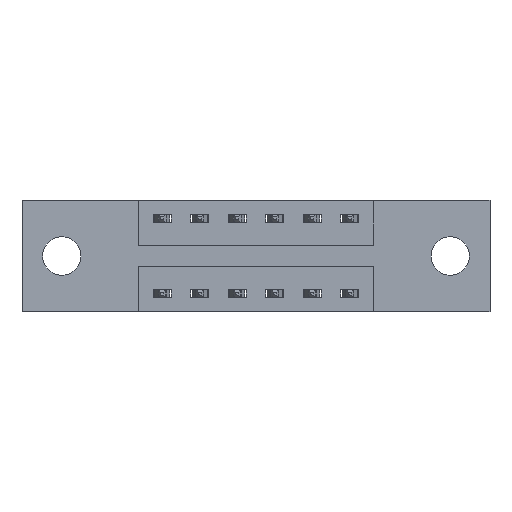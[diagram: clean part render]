
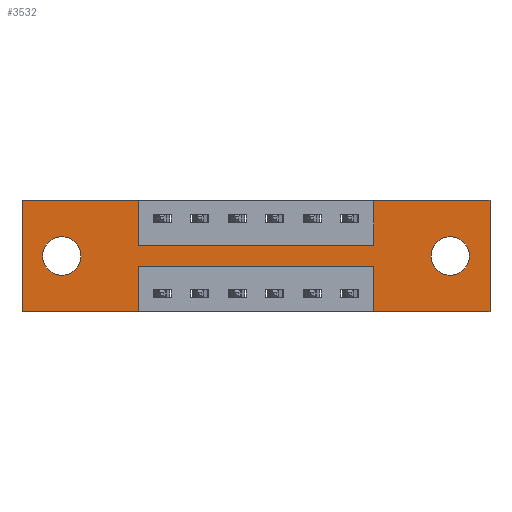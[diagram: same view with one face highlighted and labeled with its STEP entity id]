
A CAD part, front view. The second image highlights one B-rep face of the part: STEP entity #3532.
In plain terms, the highlighted planar face has unit normal (0, -1, 0).
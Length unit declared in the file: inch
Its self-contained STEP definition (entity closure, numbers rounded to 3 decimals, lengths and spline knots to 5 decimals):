
#54 = CARTESIAN_POINT ( 'NONE',  ( 1.1725, 0., 0. ) ) ;
#122 = EDGE_CURVE ( 'NONE', #3930, #1877, #3443, .T. ) ;
#149 = ORIENTED_EDGE ( 'NONE', *, *, #7531, .F. ) ;
#158 = FACE_BOUND ( 'NONE', #3052, .T. ) ;
#201 = CARTESIAN_POINT ( 'NONE',  ( 0.3875, 0., -0.37 ) ) ;
#232 = DIRECTION ( 'NONE',  ( 0., 0., -1. ) ) ;
#447 = CARTESIAN_POINT ( 'NONE',  ( 0.3875, 0., -0.15 ) ) ;
#563 = EDGE_CURVE ( 'NONE', #3608, #4599, #3827, .T. ) ;
#710 = EDGE_CURVE ( 'NONE', #7500, #4958, #1879, .T. ) ;
#736 = CARTESIAN_POINT ( 'NONE',  ( 0.1325, 0., -0.185 ) ) ;
#874 = CARTESIAN_POINT ( 'NONE',  ( 0.3875, 0., -0.37 ) ) ;
#875 = EDGE_LOOP ( 'NONE', ( #5387, #1862 ) ) ;
#930 = DIRECTION ( 'NONE',  ( 0., 1., 0. ) ) ;
#934 = ORIENTED_EDGE ( 'NONE', *, *, #122, .F. ) ;
#943 = CARTESIAN_POINT ( 'NONE',  ( 1.1725, 0., 0. ) ) ;
#975 = DIRECTION ( 'NONE',  ( 0., 0., 1. ) ) ;
#987 = EDGE_CURVE ( 'NONE', #2723, #8074, #1295, .T. ) ;
#1089 = CARTESIAN_POINT ( 'NONE',  ( 1.1725, 0., -0.22 ) ) ;
#1115 = DIRECTION ( 'NONE',  ( -1., 0., 0. ) ) ;
#1132 = CARTESIAN_POINT ( 'NONE',  ( 0.3875, 0., -0.15 ) ) ;
#1185 = DIRECTION ( 'NONE',  ( 0., 1., 0. ) ) ;
#1205 = FACE_OUTER_BOUND ( 'NONE', #2938, .T. ) ;
#1295 = CIRCLE ( 'NONE', #5872, 0.064 ) ;
#1348 = CARTESIAN_POINT ( 'NONE',  ( 1.56, 0., 0. ) ) ;
#1466 = CARTESIAN_POINT ( 'NONE',  ( 1.56, 0., 0. ) ) ;
#1506 = DIRECTION ( 'NONE',  ( 0., 0., 1. ) ) ;
#1535 = ORIENTED_EDGE ( 'NONE', *, *, #3470, .F. ) ;
#1571 = LINE ( 'NONE', #2842, #8649 ) ;
#1597 = ORIENTED_EDGE ( 'NONE', *, *, #1725, .F. ) ;
#1670 = LINE ( 'NONE', #1348, #3299 ) ;
#1725 = EDGE_CURVE ( 'NONE', #1744, #5013, #3434, .T. ) ;
#1727 = ORIENTED_EDGE ( 'NONE', *, *, #6704, .T. ) ;
#1744 = VERTEX_POINT ( 'NONE', #1089 ) ;
#1850 = DIRECTION ( 'NONE',  ( 0., 0., 1. ) ) ;
#1862 = ORIENTED_EDGE ( 'NONE', *, *, #987, .T. ) ;
#1877 = VERTEX_POINT ( 'NONE', #54 ) ;
#1879 = LINE ( 'NONE', #2483, #5286 ) ;
#1973 = DIRECTION ( 'NONE',  ( 0., 0., -1. ) ) ;
#2043 = VECTOR ( 'NONE', #975, 39.37008 ) ;
#2158 = DIRECTION ( 'NONE',  ( 0., 1., 0. ) ) ;
#2483 = CARTESIAN_POINT ( 'NONE',  ( 0., 0., -0.37 ) ) ;
#2507 = CIRCLE ( 'NONE', #7711, 0.064 ) ;
#2621 = ORIENTED_EDGE ( 'NONE', *, *, #5609, .F. ) ;
#2702 = VERTEX_POINT ( 'NONE', #1466 ) ;
#2723 = VERTEX_POINT ( 'NONE', #4312 ) ;
#2786 = VERTEX_POINT ( 'NONE', #7354 ) ;
#2824 = CARTESIAN_POINT ( 'NONE',  ( 1.1725, 0., -0.15 ) ) ;
#2842 = CARTESIAN_POINT ( 'NONE',  ( 0., 0., -0.37 ) ) ;
#2938 = EDGE_LOOP ( 'NONE', ( #149, #1597, #3492, #8532, #5949, #7988, #934, #2621, #7789, #4597, #1535, #4607 ) ) ;
#2948 = DIRECTION ( 'NONE',  ( 0., -1., 0. ) ) ;
#2968 = CARTESIAN_POINT ( 'NONE',  ( 0.1325, 0., -0.185 ) ) ;
#2998 = DIRECTION ( 'NONE',  ( 1., 0., 0. ) ) ;
#3052 = EDGE_LOOP ( 'NONE', ( #1727, #6418 ) ) ;
#3110 = VECTOR ( 'NONE', #1115, 39.37008 ) ;
#3230 = CARTESIAN_POINT ( 'NONE',  ( 1.1725, 0., -0.37 ) ) ;
#3299 = VECTOR ( 'NONE', #1973, 39.37008 ) ;
#3317 = VECTOR ( 'NONE', #6489, 39.37008 ) ;
#3434 = LINE ( 'NONE', #7228, #3110 ) ;
#3443 = LINE ( 'NONE', #943, #2043 ) ;
#3448 = VERTEX_POINT ( 'NONE', #874 ) ;
#3470 = EDGE_CURVE ( 'NONE', #6732, #5428, #5849, .T. ) ;
#3492 = ORIENTED_EDGE ( 'NONE', *, *, #8315, .F. ) ;
#3526 = CARTESIAN_POINT ( 'NONE',  ( 0., 0., 0. ) ) ;
#3532 = ADVANCED_FACE ( 'NONE', ( #158, #4971, #1205 ), #8740, .T. ) ;
#3608 = VERTEX_POINT ( 'NONE', #3900 ) ;
#3682 = EDGE_CURVE ( 'NONE', #3448, #6732, #1571, .T. ) ;
#3748 = LINE ( 'NONE', #4977, #4910 ) ;
#3757 = CARTESIAN_POINT ( 'NONE',  ( 0.3875, 0., 0. ) ) ;
#3827 = LINE ( 'NONE', #3757, #3317 ) ;
#3900 = CARTESIAN_POINT ( 'NONE',  ( 0.3875, 0., 0. ) ) ;
#3930 = VERTEX_POINT ( 'NONE', #2824 ) ;
#3963 = CARTESIAN_POINT ( 'NONE',  ( 1.4275, 0., -0.185 ) ) ;
#4092 = CARTESIAN_POINT ( 'NONE',  ( 0.1325, 0., -0.121 ) ) ;
#4107 = CARTESIAN_POINT ( 'NONE',  ( 0., 0., 0. ) ) ;
#4141 = DIRECTION ( 'NONE',  ( 1., 0., 0. ) ) ;
#4197 = VECTOR ( 'NONE', #6629, 39.37008 ) ;
#4231 = DIRECTION ( 'NONE',  ( -1., 0., 0. ) ) ;
#4267 = DIRECTION ( 'NONE',  ( 0., 0., -1. ) ) ;
#4312 = CARTESIAN_POINT ( 'NONE',  ( 0.1325, 0., -0.249 ) ) ;
#4468 = DIRECTION ( 'NONE',  ( -1., 0., 0. ) ) ;
#4575 = CARTESIAN_POINT ( 'NONE',  ( 1.4275, 0., -0.185 ) ) ;
#4597 = ORIENTED_EDGE ( 'NONE', *, *, #8227, .F. ) ;
#4599 = VERTEX_POINT ( 'NONE', #1132 ) ;
#4607 = ORIENTED_EDGE ( 'NONE', *, *, #3682, .F. ) ;
#4642 = VECTOR ( 'NONE', #1850, 39.37008 ) ;
#4688 = LINE ( 'NONE', #4107, #6609 ) ;
#4785 = CIRCLE ( 'NONE', #6433, 0.064 ) ;
#4834 = LINE ( 'NONE', #447, #4197 ) ;
#4910 = VECTOR ( 'NONE', #2998, 39.37008 ) ;
#4958 = VERTEX_POINT ( 'NONE', #7833 ) ;
#4971 = FACE_BOUND ( 'NONE', #875, .T. ) ;
#4977 = CARTESIAN_POINT ( 'NONE',  ( 0., 0., 0. ) ) ;
#4994 = VECTOR ( 'NONE', #6017, 39.37008 ) ;
#5001 = DIRECTION ( 'NONE',  ( 0., 0., 1. ) ) ;
#5013 = VERTEX_POINT ( 'NONE', #6687 ) ;
#5286 = VECTOR ( 'NONE', #4468, 39.37008 ) ;
#5386 = CARTESIAN_POINT ( 'NONE',  ( 1.4275, 0., -0.249 ) ) ;
#5387 = ORIENTED_EDGE ( 'NONE', *, *, #7855, .T. ) ;
#5428 = VERTEX_POINT ( 'NONE', #3526 ) ;
#5432 = CARTESIAN_POINT ( 'NONE',  ( 0., 0., -0.37 ) ) ;
#5609 = EDGE_CURVE ( 'NONE', #4599, #3930, #4834, .T. ) ;
#5849 = LINE ( 'NONE', #7232, #4642 ) ;
#5872 = AXIS2_PLACEMENT_3D ( 'NONE', #2968, #930, #5001 ) ;
#5949 = ORIENTED_EDGE ( 'NONE', *, *, #8379, .F. ) ;
#5965 = AXIS2_PLACEMENT_3D ( 'NONE', #736, #2158, #1506 ) ;
#6017 = DIRECTION ( 'NONE',  ( 0., 0., 1. ) ) ;
#6057 = LINE ( 'NONE', #201, #6175 ) ;
#6151 = CIRCLE ( 'NONE', #5965, 0.064 ) ;
#6164 = LINE ( 'NONE', #3230, #4994 ) ;
#6175 = VECTOR ( 'NONE', #4267, 39.37008 ) ;
#6418 = ORIENTED_EDGE ( 'NONE', *, *, #7483, .T. ) ;
#6433 = AXIS2_PLACEMENT_3D ( 'NONE', #3963, #8642, #8665 ) ;
#6489 = DIRECTION ( 'NONE',  ( 0., 0., -1. ) ) ;
#6609 = VECTOR ( 'NONE', #4141, 39.37008 ) ;
#6629 = DIRECTION ( 'NONE',  ( 1., 0., 0. ) ) ;
#6687 = CARTESIAN_POINT ( 'NONE',  ( 0.3875, 0., -0.22 ) ) ;
#6704 = EDGE_CURVE ( 'NONE', #2786, #8386, #2507, .T. ) ;
#6732 = VERTEX_POINT ( 'NONE', #5432 ) ;
#7076 = CARTESIAN_POINT ( 'NONE',  ( 0., 0., -0.37 ) ) ;
#7164 = DIRECTION ( 'NONE',  ( 0., 0., -1. ) ) ;
#7228 = CARTESIAN_POINT ( 'NONE',  ( 0.3875, 0., -0.22 ) ) ;
#7232 = CARTESIAN_POINT ( 'NONE',  ( 0., 0., 0. ) ) ;
#7354 = CARTESIAN_POINT ( 'NONE',  ( 1.4275, 0., -0.121 ) ) ;
#7398 = CARTESIAN_POINT ( 'NONE',  ( 1.56, 0., -0.37 ) ) ;
#7483 = EDGE_CURVE ( 'NONE', #8386, #2786, #4785, .T. ) ;
#7500 = VERTEX_POINT ( 'NONE', #7398 ) ;
#7531 = EDGE_CURVE ( 'NONE', #5013, #3448, #6057, .T. ) ;
#7646 = EDGE_CURVE ( 'NONE', #1877, #2702, #4688, .T. ) ;
#7711 = AXIS2_PLACEMENT_3D ( 'NONE', #4575, #1185, #7164 ) ;
#7789 = ORIENTED_EDGE ( 'NONE', *, *, #563, .F. ) ;
#7833 = CARTESIAN_POINT ( 'NONE',  ( 1.1725, 0., -0.37 ) ) ;
#7855 = EDGE_CURVE ( 'NONE', #8074, #2723, #6151, .T. ) ;
#7988 = ORIENTED_EDGE ( 'NONE', *, *, #7646, .F. ) ;
#8074 = VERTEX_POINT ( 'NONE', #4092 ) ;
#8227 = EDGE_CURVE ( 'NONE', #5428, #3608, #3748, .T. ) ;
#8315 = EDGE_CURVE ( 'NONE', #4958, #1744, #6164, .T. ) ;
#8379 = EDGE_CURVE ( 'NONE', #2702, #7500, #1670, .T. ) ;
#8386 = VERTEX_POINT ( 'NONE', #5386 ) ;
#8532 = ORIENTED_EDGE ( 'NONE', *, *, #710, .F. ) ;
#8627 = AXIS2_PLACEMENT_3D ( 'NONE', #7076, #2948, #232 ) ;
#8642 = DIRECTION ( 'NONE',  ( 0., 1., 0. ) ) ;
#8649 = VECTOR ( 'NONE', #4231, 39.37008 ) ;
#8665 = DIRECTION ( 'NONE',  ( 0., 0., -1. ) ) ;
#8740 = PLANE ( 'NONE',  #8627 ) ;
